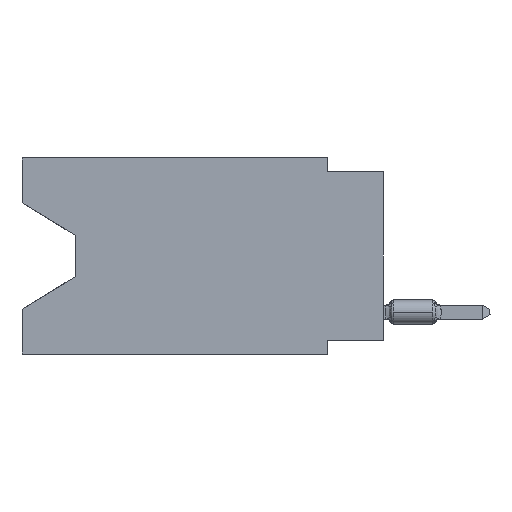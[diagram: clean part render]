
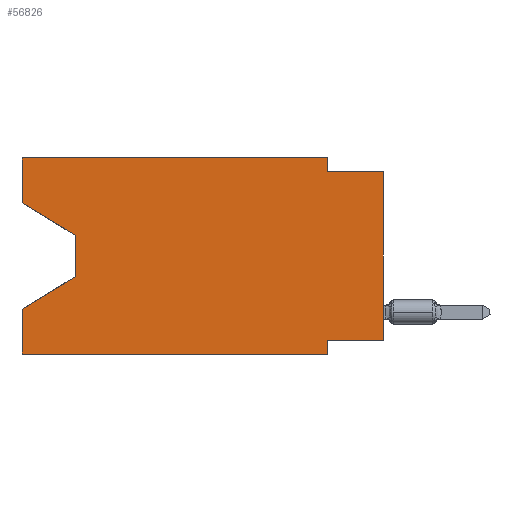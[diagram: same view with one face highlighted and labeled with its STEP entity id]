
A CAD part, left-side view. The second image highlights one B-rep face of the part: STEP entity #56826.
In plain terms, the highlighted planar face has unit normal (-1, 0, 0).
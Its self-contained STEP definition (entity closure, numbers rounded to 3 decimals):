
#2233 = CARTESIAN_POINT ( 'NONE',  ( 0., 16.383, -2.038 ) ) ;
#3032 = CARTESIAN_POINT ( 'NONE',  ( 0., 13.97, -5.385 ) ) ;
#4033 = PLANE ( 'NONE',  #20407 ) ;
#4130 = DIRECTION ( 'NONE',  ( 0., -1., 0. ) ) ;
#5770 = ORIENTED_EDGE ( 'NONE', *, *, #91867, .F. ) ;
#6127 = VERTEX_POINT ( 'NONE', #59523 ) ;
#7859 = DIRECTION ( 'NONE',  ( 0., 0., 1. ) ) ;
#10041 = EDGE_CURVE ( 'NONE', #72562, #70729, #48470, .T. ) ;
#11905 = DIRECTION ( 'NONE',  ( 0., 0., 1. ) ) ;
#12448 = ORIENTED_EDGE ( 'NONE', *, *, #58581, .F. ) ;
#12483 = ORIENTED_EDGE ( 'NONE', *, *, #19867, .F. ) ;
#13651 = VERTEX_POINT ( 'NONE', #91806 ) ;
#13774 = VECTOR ( 'NONE', #96016, 1000. ) ;
#14895 = VERTEX_POINT ( 'NONE', #23921 ) ;
#15341 = VECTOR ( 'NONE', #11905, 1000. ) ;
#16359 = ORIENTED_EDGE ( 'NONE', *, *, #41000, .T. ) ;
#19179 = DIRECTION ( 'NONE',  ( 1., 0., 0. ) ) ;
#19867 = EDGE_CURVE ( 'NONE', #71983, #46896, #88999, .T. ) ;
#20407 = AXIS2_PLACEMENT_3D ( 'NONE', #56797, #19179, #93916 ) ;
#20655 = VECTOR ( 'NONE', #75176, 1000. ) ;
#20779 = CARTESIAN_POINT ( 'NONE',  ( 0., 2.54, -8.89 ) ) ;
#21453 = LINE ( 'NONE', #72293, #78403 ) ;
#21943 = ORIENTED_EDGE ( 'NONE', *, *, #83756, .F. ) ;
#23921 = CARTESIAN_POINT ( 'NONE',  ( 0., 16.383, 0. ) ) ;
#23944 = CARTESIAN_POINT ( 'NONE',  ( 0., 16.383, -6.852 ) ) ;
#24005 = EDGE_LOOP ( 'NONE', ( #55172, #16359, #74637, #12448, #65620, #88338, #91818, #43677, #12483, #90849, #21943, #5770 ) ) ;
#24188 = CARTESIAN_POINT ( 'NONE',  ( 0., 16.383, -8.89 ) ) ;
#24738 = CARTESIAN_POINT ( 'NONE',  ( 0., 0., -8.255 ) ) ;
#25029 = EDGE_CURVE ( 'NONE', #50238, #68616, #77274, .T. ) ;
#26421 = DIRECTION ( 'NONE',  ( 0., -0.855, -0.519 ) ) ;
#28923 = CARTESIAN_POINT ( 'NONE',  ( 0., 13.97, -3.505 ) ) ;
#29077 = CARTESIAN_POINT ( 'NONE',  ( 0., 0., -8.255 ) ) ;
#29380 = CARTESIAN_POINT ( 'NONE',  ( 0., 0., 0. ) ) ;
#29402 = CARTESIAN_POINT ( 'NONE',  ( 0., 0., -0.635 ) ) ;
#30357 = VECTOR ( 'NONE', #32505, 1000. ) ;
#30537 = LINE ( 'NONE', #29077, #13774 ) ;
#30950 = CARTESIAN_POINT ( 'NONE',  ( 0., 2.54, -0.635 ) ) ;
#32420 = VECTOR ( 'NONE', #80716, 1000. ) ;
#32505 = DIRECTION ( 'NONE',  ( 0., -1., 0. ) ) ;
#32544 = EDGE_CURVE ( 'NONE', #55164, #13651, #52055, .T. ) ;
#32563 = EDGE_CURVE ( 'NONE', #62394, #55164, #30537, .T. ) ;
#34314 = FACE_OUTER_BOUND ( 'NONE', #24005, .T. ) ;
#34862 = CARTESIAN_POINT ( 'NONE',  ( 0., 16.383, 0. ) ) ;
#35980 = CARTESIAN_POINT ( 'NONE',  ( 0., 13.97, -3.505 ) ) ;
#36123 = DIRECTION ( 'NONE',  ( 0., 0., 1. ) ) ;
#40800 = LINE ( 'NONE', #34862, #15341 ) ;
#41000 = EDGE_CURVE ( 'NONE', #68616, #72562, #86590, .T. ) ;
#43074 = CARTESIAN_POINT ( 'NONE',  ( 0., 2.54, -8.255 ) ) ;
#43677 = ORIENTED_EDGE ( 'NONE', *, *, #64799, .T. ) ;
#46896 = VERTEX_POINT ( 'NONE', #69787 ) ;
#47535 = CARTESIAN_POINT ( 'NONE',  ( 0., 16.383, -8.89 ) ) ;
#48470 = LINE ( 'NONE', #3032, #61344 ) ;
#50238 = VERTEX_POINT ( 'NONE', #2233 ) ;
#51506 = VECTOR ( 'NONE', #75801, 1000. ) ;
#52055 = LINE ( 'NONE', #20779, #88681 ) ;
#55164 = VERTEX_POINT ( 'NONE', #43074 ) ;
#55172 = ORIENTED_EDGE ( 'NONE', *, *, #25029, .T. ) ;
#56797 = CARTESIAN_POINT ( 'NONE',  ( 0., 16.383, 0. ) ) ;
#56826 = ADVANCED_FACE ( 'NONE', ( #34314 ), #4033, .F. ) ;
#58581 = EDGE_CURVE ( 'NONE', #92271, #70729, #21453, .T. ) ;
#59523 = CARTESIAN_POINT ( 'NONE',  ( 0., 2.54, 0. ) ) ;
#60141 = VECTOR ( 'NONE', #4130, 1000. ) ;
#61344 = VECTOR ( 'NONE', #71403, 1000. ) ;
#62394 = VERTEX_POINT ( 'NONE', #24738 ) ;
#62560 = VECTOR ( 'NONE', #26421, 1000. ) ;
#64222 = CARTESIAN_POINT ( 'NONE',  ( 0., 16.383, 0. ) ) ;
#64799 = EDGE_CURVE ( 'NONE', #62394, #46896, #74815, .T. ) ;
#65180 = LINE ( 'NONE', #64222, #60141 ) ;
#65620 = ORIENTED_EDGE ( 'NONE', *, *, #82341, .T. ) ;
#65796 = CARTESIAN_POINT ( 'NONE',  ( 0., 13.97, -5.385 ) ) ;
#68616 = VERTEX_POINT ( 'NONE', #35980 ) ;
#68823 = CARTESIAN_POINT ( 'NONE',  ( 0., 2.54, 0. ) ) ;
#69787 = CARTESIAN_POINT ( 'NONE',  ( 0., 0., -0.635 ) ) ;
#70729 = VERTEX_POINT ( 'NONE', #23944 ) ;
#71403 = DIRECTION ( 'NONE',  ( 0., 0.855, -0.519 ) ) ;
#71983 = VERTEX_POINT ( 'NONE', #30950 ) ;
#72293 = CARTESIAN_POINT ( 'NONE',  ( 0., 16.383, 0. ) ) ;
#72407 = EDGE_CURVE ( 'NONE', #6127, #71983, #89810, .T. ) ;
#72562 = VERTEX_POINT ( 'NONE', #65796 ) ;
#74637 = ORIENTED_EDGE ( 'NONE', *, *, #10041, .T. ) ;
#74815 = LINE ( 'NONE', #29380, #76011 ) ;
#75176 = DIRECTION ( 'NONE',  ( 0., 0., -1. ) ) ;
#75801 = DIRECTION ( 'NONE',  ( 0., -1., 0. ) ) ;
#76011 = VECTOR ( 'NONE', #7859, 1000. ) ;
#77274 = LINE ( 'NONE', #86036, #62560 ) ;
#78403 = VECTOR ( 'NONE', #36123, 1000. ) ;
#80716 = DIRECTION ( 'NONE',  ( 0., 0., -1. ) ) ;
#82341 = EDGE_CURVE ( 'NONE', #92271, #13651, #84772, .T. ) ;
#83756 = EDGE_CURVE ( 'NONE', #14895, #6127, #65180, .T. ) ;
#84772 = LINE ( 'NONE', #24188, #30357 ) ;
#86036 = CARTESIAN_POINT ( 'NONE',  ( 0., 16.383, -2.038 ) ) ;
#86590 = LINE ( 'NONE', #28923, #32420 ) ;
#87709 = DIRECTION ( 'NONE',  ( 0., 0., -1. ) ) ;
#88338 = ORIENTED_EDGE ( 'NONE', *, *, #32544, .F. ) ;
#88681 = VECTOR ( 'NONE', #87709, 1000. ) ;
#88999 = LINE ( 'NONE', #29402, #51506 ) ;
#89810 = LINE ( 'NONE', #68823, #20655 ) ;
#90849 = ORIENTED_EDGE ( 'NONE', *, *, #72407, .F. ) ;
#91806 = CARTESIAN_POINT ( 'NONE',  ( 0., 2.54, -8.89 ) ) ;
#91818 = ORIENTED_EDGE ( 'NONE', *, *, #32563, .F. ) ;
#91867 = EDGE_CURVE ( 'NONE', #50238, #14895, #40800, .T. ) ;
#92271 = VERTEX_POINT ( 'NONE', #47535 ) ;
#93916 = DIRECTION ( 'NONE',  ( 0., 0., -1. ) ) ;
#96016 = DIRECTION ( 'NONE',  ( 0., 1., 0. ) ) ;
